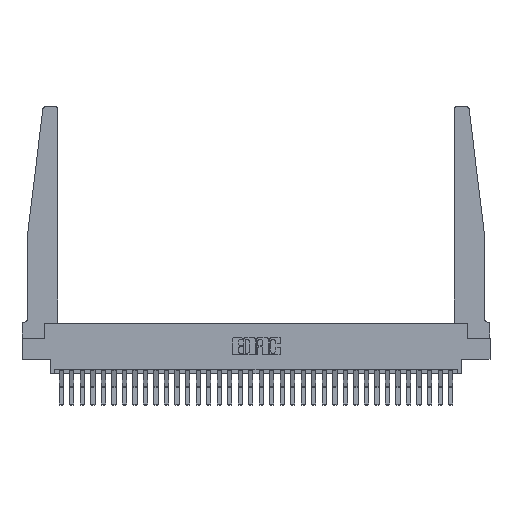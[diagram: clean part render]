
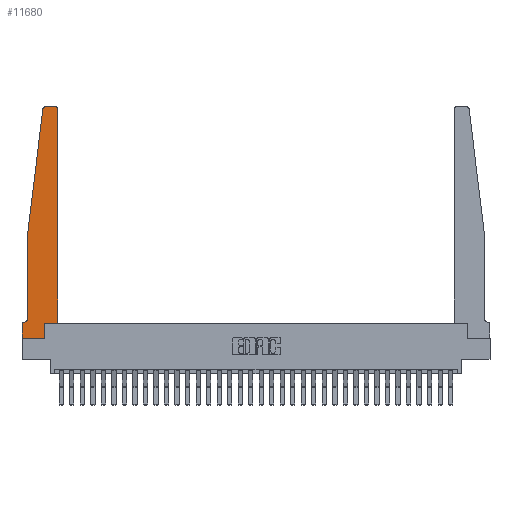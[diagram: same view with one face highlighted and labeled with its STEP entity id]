
A CAD part, top view. The second image highlights one B-rep face of the part: STEP entity #11680.
In plain terms, the highlighted planar face has unit normal (0, 0, 1).
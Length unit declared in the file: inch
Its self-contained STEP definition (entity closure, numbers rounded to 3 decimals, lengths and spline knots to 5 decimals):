
#810 = CARTESIAN_POINT ( 'NONE',  ( 0.065, 1.25, 0.37 ) ) ;
#813 = ORIENTED_EDGE ( 'NONE', *, *, #14321, .T. ) ;
#815 = CARTESIAN_POINT ( 'NONE',  ( 0., 0.1875, 0.37 ) ) ;
#965 = DIRECTION ( 'NONE',  ( -0.122, -0.992, 0. ) ) ;
#2307 = CARTESIAN_POINT ( 'NONE',  ( 0.2605, 0., 0.37 ) ) ;
#2411 = CARTESIAN_POINT ( 'NONE',  ( 0., 0., 0.37 ) ) ;
#2665 = VECTOR ( 'NONE', #22900, 39.37008 ) ;
#3015 = FACE_OUTER_BOUND ( 'NONE', #13138, .T. ) ;
#3123 = LINE ( 'NONE', #26351, #30560 ) ;
#3182 = DIRECTION ( 'NONE',  ( 0., -1., 0. ) ) ;
#3469 = CARTESIAN_POINT ( 'NONE',  ( 0.25, 2.75, 0.37 ) ) ;
#3941 = DIRECTION ( 'NONE',  ( -1., 0., 0. ) ) ;
#4115 = DIRECTION ( 'NONE',  ( 1., 0., 0. ) ) ;
#4226 = VERTEX_POINT ( 'NONE', #10367 ) ;
#4340 = ORIENTED_EDGE ( 'NONE', *, *, #13243, .T. ) ;
#4724 = CARTESIAN_POINT ( 'NONE',  ( 0.425, 0.18, 0.37 ) ) ;
#4856 = ORIENTED_EDGE ( 'NONE', *, *, #12099, .T. ) ;
#4904 = VECTOR ( 'NONE', #3182, 39.37008 ) ;
#5015 = CARTESIAN_POINT ( 'NONE',  ( 0.24675, 2.72367, 0.37 ) ) ;
#5129 = EDGE_CURVE ( 'NONE', #8436, #15493, #10663, .T. ) ;
#5602 = EDGE_CURVE ( 'NONE', #15493, #20459, #14314, .T. ) ;
#6234 = CARTESIAN_POINT ( 'NONE',  ( 0.065, 1.25, 0.37 ) ) ;
#6448 = VERTEX_POINT ( 'NONE', #20495 ) ;
#6464 = ORIENTED_EDGE ( 'NONE', *, *, #28800, .T. ) ;
#6547 = CARTESIAN_POINT ( 'NONE',  ( 0.2605, 0.18, 0.37 ) ) ;
#7046 = LINE ( 'NONE', #9383, #20273 ) ;
#7209 = VECTOR ( 'NONE', #21751, 39.37008 ) ;
#7415 = VERTEX_POINT ( 'NONE', #11348 ) ;
#8343 = AXIS2_PLACEMENT_3D ( 'NONE', #16037, #20569, #18375 ) ;
#8381 = EDGE_CURVE ( 'NONE', #13792, #12759, #26072, .T. ) ;
#8436 = VERTEX_POINT ( 'NONE', #6234 ) ;
#8624 = VERTEX_POINT ( 'NONE', #27609 ) ;
#9089 = EDGE_CURVE ( 'NONE', #17121, #23172, #13353, .T. ) ;
#9383 = CARTESIAN_POINT ( 'NONE',  ( 0.425, 0.18, 0.37 ) ) ;
#10127 = CARTESIAN_POINT ( 'NONE',  ( 0.395, 2.72, 0.37 ) ) ;
#10157 = EDGE_CURVE ( 'NONE', #20459, #6448, #3123, .T. ) ;
#10164 = DIRECTION ( 'NONE',  ( 1., 0., 0. ) ) ;
#10367 = CARTESIAN_POINT ( 'NONE',  ( 0.27653, 2.75, 0.37 ) ) ;
#10471 = PLANE ( 'NONE',  #12194 ) ;
#10663 = LINE ( 'NONE', #22361, #23790 ) ;
#10782 = LINE ( 'NONE', #3469, #25895 ) ;
#10866 = ORIENTED_EDGE ( 'NONE', *, *, #9089, .T. ) ;
#11040 = EDGE_CURVE ( 'NONE', #23172, #13792, #26730, .T. ) ;
#11048 = ORIENTED_EDGE ( 'NONE', *, *, #16507, .T. ) ;
#11348 = CARTESIAN_POINT ( 'NONE',  ( 0.425, 2.72, 0.37 ) ) ;
#11680 = ADVANCED_FACE ( 'NONE', ( #3015 ), #10471, .T. ) ;
#12099 = EDGE_CURVE ( 'NONE', #7415, #8624, #16685, .T. ) ;
#12194 = AXIS2_PLACEMENT_3D ( 'NONE', #815, #19971, #10164 ) ;
#12365 = DIRECTION ( 'NONE',  ( 1., 0., 0. ) ) ;
#12759 = VERTEX_POINT ( 'NONE', #25325 ) ;
#13138 = EDGE_LOOP ( 'NONE', ( #6464, #813, #4340, #18177, #26898, #20330, #21457, #10866, #16323, #17394, #11048, #4856 ) ) ;
#13216 = LINE ( 'NONE', #17331, #4904 ) ;
#13243 = EDGE_CURVE ( 'NONE', #18918, #8436, #26538, .T. ) ;
#13353 = LINE ( 'NONE', #19928, #2665 ) ;
#13792 = VERTEX_POINT ( 'NONE', #6547 ) ;
#14314 = CIRCLE ( 'NONE', #8343, 0.05 ) ;
#14321 = EDGE_CURVE ( 'NONE', #4226, #18918, #14691, .T. ) ;
#14691 = CIRCLE ( 'NONE', #18708, 0.03 ) ;
#15493 = VERTEX_POINT ( 'NONE', #25838 ) ;
#15831 = DIRECTION ( 'NONE',  ( 1., 0., 0. ) ) ;
#16037 = CARTESIAN_POINT ( 'NONE',  ( 0.015, 0.2375, 0.37 ) ) ;
#16323 = ORIENTED_EDGE ( 'NONE', *, *, #11040, .T. ) ;
#16507 = EDGE_CURVE ( 'NONE', #12759, #7415, #7046, .T. ) ;
#16685 = CIRCLE ( 'NONE', #23697, 0.03 ) ;
#17121 = VERTEX_POINT ( 'NONE', #2411 ) ;
#17331 = CARTESIAN_POINT ( 'NONE',  ( 0., 0., 0.37 ) ) ;
#17394 = ORIENTED_EDGE ( 'NONE', *, *, #8381, .T. ) ;
#18177 = ORIENTED_EDGE ( 'NONE', *, *, #5129, .T. ) ;
#18221 = CARTESIAN_POINT ( 'NONE',  ( 0.015, 0.1875, 0.37 ) ) ;
#18375 = DIRECTION ( 'NONE',  ( -1., 0., 0. ) ) ;
#18708 = AXIS2_PLACEMENT_3D ( 'NONE', #29074, #21452, #12365 ) ;
#18893 = VECTOR ( 'NONE', #4115, 39.37008 ) ;
#18918 = VERTEX_POINT ( 'NONE', #5015 ) ;
#19756 = DIRECTION ( 'NONE',  ( 0., 1., 0. ) ) ;
#19928 = CARTESIAN_POINT ( 'NONE',  ( 0., 0., 0.37 ) ) ;
#19971 = DIRECTION ( 'NONE',  ( 0., 0., 1. ) ) ;
#20273 = VECTOR ( 'NONE', #19756, 39.37008 ) ;
#20330 = ORIENTED_EDGE ( 'NONE', *, *, #10157, .T. ) ;
#20459 = VERTEX_POINT ( 'NONE', #18221 ) ;
#20495 = CARTESIAN_POINT ( 'NONE',  ( 0., 0.1875, 0.37 ) ) ;
#20569 = DIRECTION ( 'NONE',  ( 0., 0., -1. ) ) ;
#21452 = DIRECTION ( 'NONE',  ( 0., 0., 1. ) ) ;
#21457 = ORIENTED_EDGE ( 'NONE', *, *, #24648, .T. ) ;
#21751 = DIRECTION ( 'NONE',  ( 0., 1., 0. ) ) ;
#22361 = CARTESIAN_POINT ( 'NONE',  ( 0.065, 1.25, 0.37 ) ) ;
#22723 = VECTOR ( 'NONE', #965, 39.37008 ) ;
#22900 = DIRECTION ( 'NONE',  ( 1., 0., 0. ) ) ;
#23172 = VERTEX_POINT ( 'NONE', #2307 ) ;
#23697 = AXIS2_PLACEMENT_3D ( 'NONE', #10127, #27702, #15831 ) ;
#23790 = VECTOR ( 'NONE', #29839, 39.37008 ) ;
#24176 = DIRECTION ( 'NONE',  ( -1., 0., 0. ) ) ;
#24648 = EDGE_CURVE ( 'NONE', #6448, #17121, #13216, .T. ) ;
#25325 = CARTESIAN_POINT ( 'NONE',  ( 0.425, 0.18, 0.37 ) ) ;
#25838 = CARTESIAN_POINT ( 'NONE',  ( 0.065, 0.2375, 0.37 ) ) ;
#25895 = VECTOR ( 'NONE', #3941, 39.37008 ) ;
#26072 = LINE ( 'NONE', #4724, #18893 ) ;
#26351 = CARTESIAN_POINT ( 'NONE',  ( 0.065, 0.1875, 0.37 ) ) ;
#26538 = LINE ( 'NONE', #810, #22723 ) ;
#26730 = LINE ( 'NONE', #28769, #7209 ) ;
#26898 = ORIENTED_EDGE ( 'NONE', *, *, #5602, .T. ) ;
#27609 = CARTESIAN_POINT ( 'NONE',  ( 0.395, 2.75, 0.37 ) ) ;
#27702 = DIRECTION ( 'NONE',  ( 0., 0., 1. ) ) ;
#28769 = CARTESIAN_POINT ( 'NONE',  ( 0.2605, 0.18, 0.37 ) ) ;
#28800 = EDGE_CURVE ( 'NONE', #8624, #4226, #10782, .T. ) ;
#29074 = CARTESIAN_POINT ( 'NONE',  ( 0.27653, 2.72, 0.37 ) ) ;
#29839 = DIRECTION ( 'NONE',  ( 0., -1., 0. ) ) ;
#30560 = VECTOR ( 'NONE', #24176, 39.37008 ) ;
